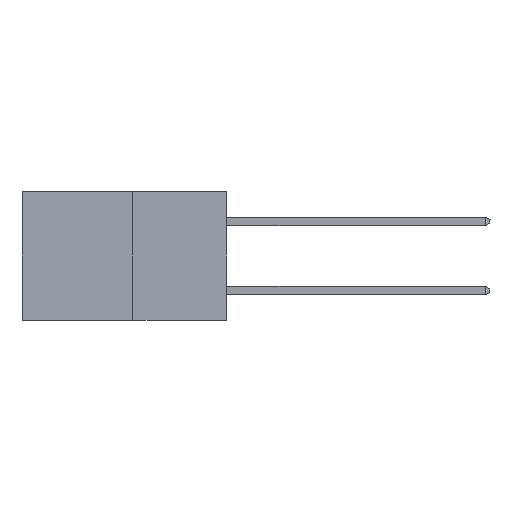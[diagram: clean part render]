
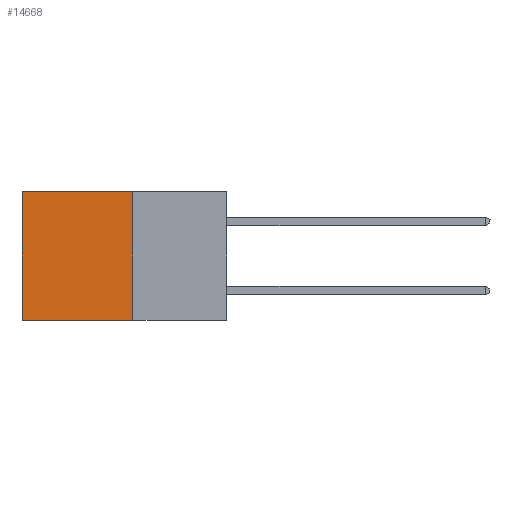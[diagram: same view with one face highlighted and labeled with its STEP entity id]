
A CAD part, left-side view. The second image highlights one B-rep face of the part: STEP entity #14668.
In plain terms, the highlighted planar face has unit normal (-1, 0, 0).
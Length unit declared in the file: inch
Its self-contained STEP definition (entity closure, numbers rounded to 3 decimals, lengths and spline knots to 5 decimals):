
#58 = DIRECTION ( 'NONE',  ( 0., 1., 0. ) ) ;
#148 = CARTESIAN_POINT ( 'NONE',  ( 0.277, 0.27, 0. ) ) ;
#210 = CARTESIAN_POINT ( 'NONE',  ( 0.277, 0.27, -0.37 ) ) ;
#795 = VECTOR ( 'NONE', #16189, 39.37008 ) ;
#2555 = CARTESIAN_POINT ( 'NONE',  ( 0.277, 0.27, 0. ) ) ;
#2612 = DIRECTION ( 'NONE',  ( 1., 0., 0. ) ) ;
#2804 = AXIS2_PLACEMENT_3D ( 'NONE', #10935, #2612, #12285 ) ;
#2947 = CARTESIAN_POINT ( 'NONE',  ( 0.277, 0.27, -0.37 ) ) ;
#3768 = VECTOR ( 'NONE', #12588, 39.37008 ) ;
#5559 = ORIENTED_EDGE ( 'NONE', *, *, #7327, .F. ) ;
#6023 = CARTESIAN_POINT ( 'NONE',  ( 0.277, 0.59, -0.37 ) ) ;
#6224 = EDGE_CURVE ( 'NONE', #11514, #15439, #16032, .T. ) ;
#6926 = ORIENTED_EDGE ( 'NONE', *, *, #6224, .T. ) ;
#7041 = ORIENTED_EDGE ( 'NONE', *, *, #12635, .T. ) ;
#7092 = LINE ( 'NONE', #2947, #3768 ) ;
#7327 = EDGE_CURVE ( 'NONE', #12358, #17443, #11871, .T. ) ;
#8235 = CARTESIAN_POINT ( 'NONE',  ( 0.277, 0.59, -0.37 ) ) ;
#8333 = CARTESIAN_POINT ( 'NONE',  ( 0.277, 0.59, 0. ) ) ;
#8522 = LINE ( 'NONE', #8235, #8958 ) ;
#8958 = VECTOR ( 'NONE', #12282, 39.37008 ) ;
#9563 = CARTESIAN_POINT ( 'NONE',  ( 0.277, 0.27, -0.37 ) ) ;
#10935 = CARTESIAN_POINT ( 'NONE',  ( 0.277, 0.27, -0.37 ) ) ;
#11049 = EDGE_LOOP ( 'NONE', ( #7041, #5559, #15575, #6926 ) ) ;
#11078 = EDGE_CURVE ( 'NONE', #11514, #12358, #7092, .T. ) ;
#11514 = VERTEX_POINT ( 'NONE', #2555 ) ;
#11871 = LINE ( 'NONE', #9563, #795 ) ;
#12282 = DIRECTION ( 'NONE',  ( 0., 0., -1. ) ) ;
#12285 = DIRECTION ( 'NONE',  ( 0., 0., -1. ) ) ;
#12358 = VERTEX_POINT ( 'NONE', #210 ) ;
#12529 = VECTOR ( 'NONE', #58, 39.37008 ) ;
#12588 = DIRECTION ( 'NONE',  ( 0., 0., -1. ) ) ;
#12635 = EDGE_CURVE ( 'NONE', #15439, #17443, #8522, .T. ) ;
#14327 = FACE_OUTER_BOUND ( 'NONE', #11049, .T. ) ;
#14668 = ADVANCED_FACE ( 'NONE', ( #14327 ), #14913, .F. ) ;
#14913 = PLANE ( 'NONE',  #2804 ) ;
#15439 = VERTEX_POINT ( 'NONE', #8333 ) ;
#15575 = ORIENTED_EDGE ( 'NONE', *, *, #11078, .F. ) ;
#16032 = LINE ( 'NONE', #148, #12529 ) ;
#16189 = DIRECTION ( 'NONE',  ( 0., 1., 0. ) ) ;
#17443 = VERTEX_POINT ( 'NONE', #6023 ) ;
